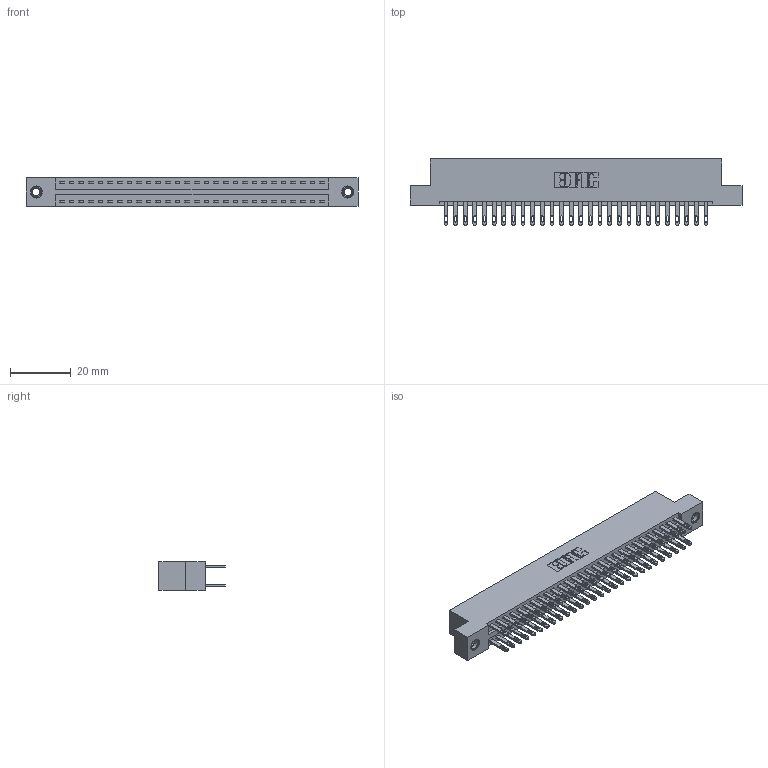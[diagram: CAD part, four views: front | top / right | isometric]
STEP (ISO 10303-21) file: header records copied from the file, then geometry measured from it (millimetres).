
FILE_DESCRIPTION (( 'STEP AP203' ), '1' );
FILE_NAME ('346-056-500-207.STEP', '2018-08-28T02:07:06', ( '' ), ( '' ), 'SwSTEP 2.0', 'SolidWorks 2016', '' );
FILE_SCHEMA (( 'CONFIG_CONTROL_DESIGN' ));
Length unit declared in the file: inch
Products named in the file (4): 346 Part_Flush Mounting Lugs - 0.156 Dia-TI; 345-292-001_345-293-100; 345-250-001_345-250-005-103; 346-056-500-207
Assembly tree (59 placements, depth 2):
  346-056-500-207
    346 Part_Flush Mounting Lugs - 0.156 Dia-TI
    345-292-001_345-293-100  x56
    345-250-001_345-250-005-103  x2
Bounding box: 109.47 x 21.84 x 9.4 mm (x, y, z)
Volume: 10723.9 mm3; surface area: 15140.6 mm2
Topology: 59 solids, 59 shells, 2870 faces, 8697 edges, 5790 vertices
Faces by surface type: plane 1732, cylinder 1122, cone 12, torus 4
Entity records: 21274 total; most frequent: CARTESIAN_POINT 3507, ORIENTED_EDGE 3434, DIRECTION 3171, EDGE_CURVE 1717, VECTOR 1449, LINE 1449, VERTEX_POINT 1140, AXIS2_PLACEMENT_3D 861
